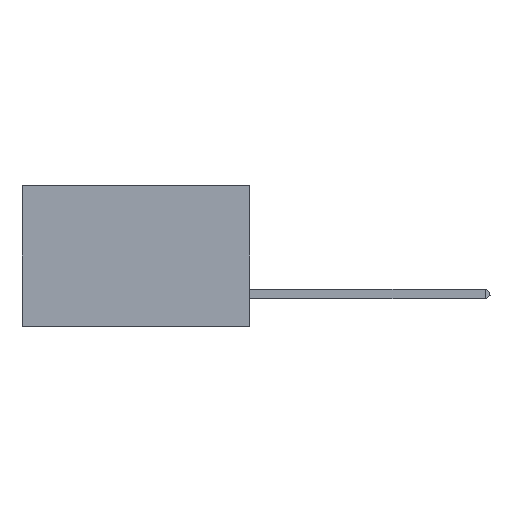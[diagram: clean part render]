
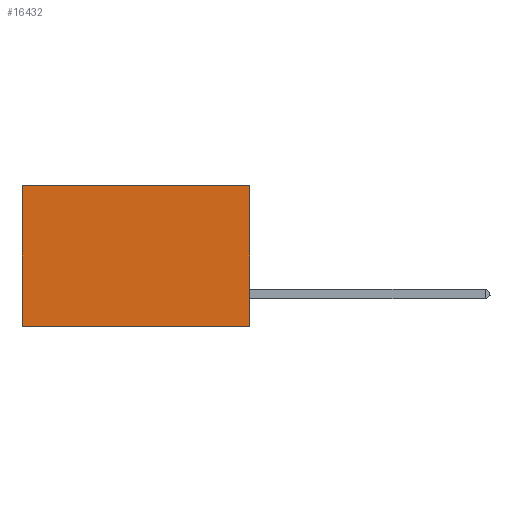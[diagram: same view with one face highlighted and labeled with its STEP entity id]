
A CAD part, left-side view. The second image highlights one B-rep face of the part: STEP entity #16432.
In plain terms, the highlighted planar face has unit normal (-1, 0, 0).
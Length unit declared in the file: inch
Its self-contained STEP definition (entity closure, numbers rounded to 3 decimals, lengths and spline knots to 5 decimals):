
#251 = ORIENTED_EDGE ( 'NONE', *, *, #5190, .T. ) ;
#583 = LINE ( 'NONE', #3138, #6205 ) ;
#893 = CARTESIAN_POINT ( 'NONE',  ( 0.2875, 0.6, -0.37 ) ) ;
#1466 = CARTESIAN_POINT ( 'NONE',  ( 0.2875, 0., 0. ) ) ;
#1555 = CARTESIAN_POINT ( 'NONE',  ( 0.2875, 0., 0. ) ) ;
#1793 = EDGE_CURVE ( 'NONE', #16033, #13054, #11423, .T. ) ;
#1938 = ORIENTED_EDGE ( 'NONE', *, *, #13821, .T. ) ;
#2196 = VECTOR ( 'NONE', #15480, 39.37008 ) ;
#2535 = CARTESIAN_POINT ( 'NONE',  ( 0.2875, 0., 0. ) ) ;
#2882 = EDGE_LOOP ( 'NONE', ( #251, #4595, #9828, #1938 ) ) ;
#3138 = CARTESIAN_POINT ( 'NONE',  ( 0.2875, 0.6, 0. ) ) ;
#3197 = EDGE_CURVE ( 'NONE', #13054, #14954, #10504, .T. ) ;
#4027 = AXIS2_PLACEMENT_3D ( 'NONE', #7956, #10670, #5036 ) ;
#4595 = ORIENTED_EDGE ( 'NONE', *, *, #3197, .F. ) ;
#5036 = DIRECTION ( 'NONE',  ( 0., 0., -1. ) ) ;
#5190 = EDGE_CURVE ( 'NONE', #17521, #14954, #583, .T. ) ;
#6205 = VECTOR ( 'NONE', #14026, 39.37008 ) ;
#7723 = CARTESIAN_POINT ( 'NONE',  ( 0.2875, 0.6, 0. ) ) ;
#7956 = CARTESIAN_POINT ( 'NONE',  ( 0.2875, 0., 0. ) ) ;
#9828 = ORIENTED_EDGE ( 'NONE', *, *, #1793, .F. ) ;
#10118 = CARTESIAN_POINT ( 'NONE',  ( 0.2875, 0., -0.37 ) ) ;
#10504 = LINE ( 'NONE', #10118, #17741 ) ;
#10670 = DIRECTION ( 'NONE',  ( 1., 0., 0. ) ) ;
#10704 = FACE_OUTER_BOUND ( 'NONE', #2882, .T. ) ;
#11381 = DIRECTION ( 'NONE',  ( 0., 1., 0. ) ) ;
#11423 = LINE ( 'NONE', #2535, #16098 ) ;
#13054 = VERTEX_POINT ( 'NONE', #13271 ) ;
#13271 = CARTESIAN_POINT ( 'NONE',  ( 0.2875, 0., -0.37 ) ) ;
#13821 = EDGE_CURVE ( 'NONE', #16033, #17521, #17218, .T. ) ;
#14026 = DIRECTION ( 'NONE',  ( 0., 0., -1. ) ) ;
#14954 = VERTEX_POINT ( 'NONE', #893 ) ;
#15480 = DIRECTION ( 'NONE',  ( 0., 1., 0. ) ) ;
#16033 = VERTEX_POINT ( 'NONE', #1466 ) ;
#16098 = VECTOR ( 'NONE', #16253, 39.37008 ) ;
#16253 = DIRECTION ( 'NONE',  ( 0., 0., -1. ) ) ;
#16432 = ADVANCED_FACE ( 'NONE', ( #10704 ), #17423, .F. ) ;
#17218 = LINE ( 'NONE', #1555, #2196 ) ;
#17423 = PLANE ( 'NONE',  #4027 ) ;
#17521 = VERTEX_POINT ( 'NONE', #7723 ) ;
#17741 = VECTOR ( 'NONE', #11381, 39.37008 ) ;
